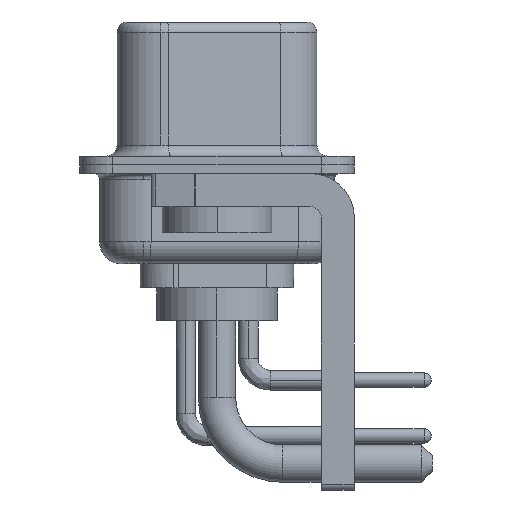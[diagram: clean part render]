
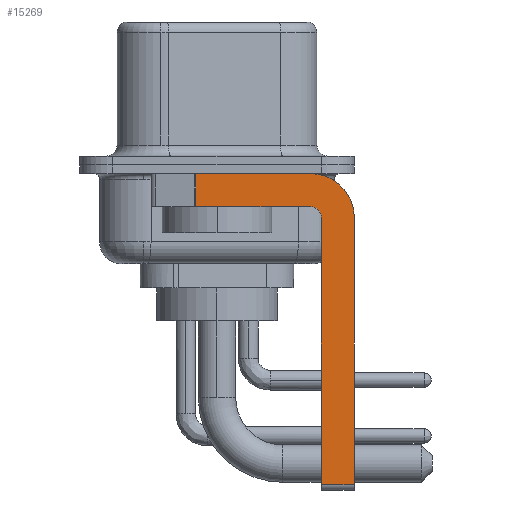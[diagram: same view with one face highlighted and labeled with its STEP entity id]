
A CAD part, left-side view. The second image highlights one B-rep face of the part: STEP entity #15269.
In plain terms, the highlighted planar face has unit normal (-1, 0, 0).
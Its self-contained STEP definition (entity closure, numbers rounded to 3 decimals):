
#214 = CARTESIAN_POINT ( 'NONE',  ( -2.9, -4.25, -2.4 ) ) ;
#220 = AXIS2_PLACEMENT_3D ( 'NONE', #214, #3585, #15100 ) ;
#313 = ORIENTED_EDGE ( 'NONE', *, *, #19952, .F. ) ;
#939 = CARTESIAN_POINT ( 'NONE',  ( -2.9, -6.25, -2.4 ) ) ;
#1902 = DIRECTION ( 'NONE',  ( 0., -1., 0. ) ) ;
#2367 = LINE ( 'NONE', #15622, #6389 ) ;
#2500 = CIRCLE ( 'NONE', #23896, 2. ) ;
#2576 = CARTESIAN_POINT ( 'NONE',  ( -2.9, 0.978, -1.9 ) ) ;
#2797 = LINE ( 'NONE', #939, #23056 ) ;
#2918 = VERTEX_POINT ( 'NONE', #19196 ) ;
#3001 = CARTESIAN_POINT ( 'NONE',  ( -2.9, -6.25, -2.4 ) ) ;
#3402 = CARTESIAN_POINT ( 'NONE',  ( -2.9, -4.25, -14.55 ) ) ;
#3585 = DIRECTION ( 'NONE',  ( -1., 0., 0. ) ) ;
#4113 = VERTEX_POINT ( 'NONE', #3001 ) ;
#4565 = DIRECTION ( 'NONE',  ( 0., 0., -1. ) ) ;
#5758 = LINE ( 'NONE', #3402, #22965 ) ;
#5792 = ORIENTED_EDGE ( 'NONE', *, *, #20231, .T. ) ;
#6110 = DIRECTION ( 'NONE',  ( 0., 0., -1. ) ) ;
#6200 = EDGE_CURVE ( 'NONE', #2918, #16071, #18403, .T. ) ;
#6389 = VECTOR ( 'NONE', #17505, 1000. ) ;
#6715 = EDGE_CURVE ( 'NONE', #14734, #2918, #21989, .T. ) ;
#7055 = ORIENTED_EDGE ( 'NONE', *, *, #10704, .T. ) ;
#7081 = CARTESIAN_POINT ( 'NONE',  ( -2.9, 3., -0.4 ) ) ;
#7767 = CARTESIAN_POINT ( 'NONE',  ( -2.9, -4.25, -2.4 ) ) ;
#9944 = CARTESIAN_POINT ( 'NONE',  ( -2.9, -6.25, -14.55 ) ) ;
#10126 = ORIENTED_EDGE ( 'NONE', *, *, #6715, .F. ) ;
#10541 = CARTESIAN_POINT ( 'NONE',  ( -2.9, 0.978, -0.4 ) ) ;
#10704 = EDGE_CURVE ( 'NONE', #14519, #22619, #5758, .T. ) ;
#10940 = CARTESIAN_POINT ( 'NONE',  ( -2.9, -4.25, -0.4 ) ) ;
#11132 = CARTESIAN_POINT ( 'NONE',  ( -2.9, -4.75, -2.4 ) ) ;
#11189 = AXIS2_PLACEMENT_3D ( 'NONE', #7767, #15300, #22883 ) ;
#12243 = CARTESIAN_POINT ( 'NONE',  ( -2.9, -4.75, -14.55 ) ) ;
#13976 = LINE ( 'NONE', #2576, #21351 ) ;
#14022 = DIRECTION ( 'NONE',  ( 1., 0., 0. ) ) ;
#14057 = CARTESIAN_POINT ( 'NONE',  ( -2.9, -4.25, -1.9 ) ) ;
#14374 = CARTESIAN_POINT ( 'NONE',  ( -2.9, 0.978, -1.9 ) ) ;
#14440 = VECTOR ( 'NONE', #18281, 1000. ) ;
#14519 = VERTEX_POINT ( 'NONE', #12243 ) ;
#14734 = VERTEX_POINT ( 'NONE', #11132 ) ;
#14738 = DIRECTION ( 'NONE',  ( 0., -1., 0. ) ) ;
#15063 = FACE_OUTER_BOUND ( 'NONE', #23291, .T. ) ;
#15100 = DIRECTION ( 'NONE',  ( 0., 0., 1. ) ) ;
#15269 = ADVANCED_FACE ( 'NONE', ( #15063 ), #16938, .F. ) ;
#15300 = DIRECTION ( 'NONE',  ( 1., 0., 0. ) ) ;
#15622 = CARTESIAN_POINT ( 'NONE',  ( -2.9, -4.75, -14.8 ) ) ;
#16001 = EDGE_CURVE ( 'NONE', #18110, #4113, #2500, .T. ) ;
#16071 = VERTEX_POINT ( 'NONE', #14374 ) ;
#16094 = VERTEX_POINT ( 'NONE', #10541 ) ;
#16475 = LINE ( 'NONE', #7081, #22120 ) ;
#16938 = PLANE ( 'NONE',  #11189 ) ;
#17138 = ORIENTED_EDGE ( 'NONE', *, *, #24369, .F. ) ;
#17505 = DIRECTION ( 'NONE',  ( 0., 0., 1. ) ) ;
#18110 = VERTEX_POINT ( 'NONE', #10940 ) ;
#18281 = DIRECTION ( 'NONE',  ( 0., 1., 0. ) ) ;
#18403 = LINE ( 'NONE', #14057, #14440 ) ;
#18765 = ORIENTED_EDGE ( 'NONE', *, *, #23373, .F. ) ;
#19196 = CARTESIAN_POINT ( 'NONE',  ( -2.9, -4.25, -1.9 ) ) ;
#19485 = CARTESIAN_POINT ( 'NONE',  ( -2.9, -4.25, -2.4 ) ) ;
#19952 = EDGE_CURVE ( 'NONE', #16094, #18110, #16475, .T. ) ;
#20231 = EDGE_CURVE ( 'NONE', #16094, #16071, #13976, .T. ) ;
#20380 = ORIENTED_EDGE ( 'NONE', *, *, #16001, .F. ) ;
#20786 = ORIENTED_EDGE ( 'NONE', *, *, #6200, .F. ) ;
#21351 = VECTOR ( 'NONE', #4565, 1000. ) ;
#21989 = CIRCLE ( 'NONE', #220, 0.5 ) ;
#22120 = VECTOR ( 'NONE', #14738, 1000. ) ;
#22619 = VERTEX_POINT ( 'NONE', #9944 ) ;
#22883 = DIRECTION ( 'NONE',  ( 0., 0., -1. ) ) ;
#22965 = VECTOR ( 'NONE', #1902, 1000. ) ;
#23056 = VECTOR ( 'NONE', #23274, 1000. ) ;
#23274 = DIRECTION ( 'NONE',  ( 0., 0., -1. ) ) ;
#23291 = EDGE_LOOP ( 'NONE', ( #313, #5792, #20786, #10126, #18765, #7055, #17138, #20380 ) ) ;
#23373 = EDGE_CURVE ( 'NONE', #14519, #14734, #2367, .T. ) ;
#23896 = AXIS2_PLACEMENT_3D ( 'NONE', #19485, #14022, #6110 ) ;
#24369 = EDGE_CURVE ( 'NONE', #4113, #22619, #2797, .T. ) ;
